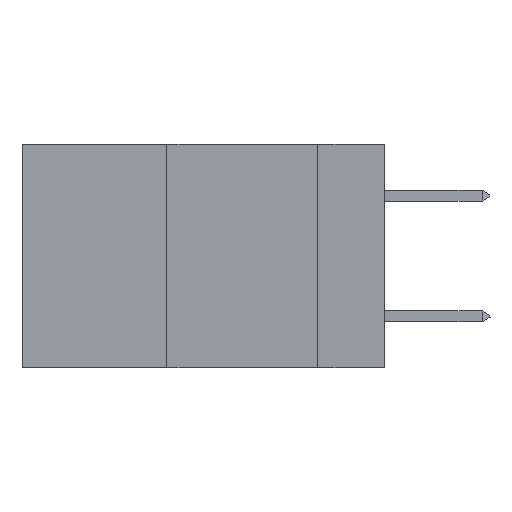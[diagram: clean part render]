
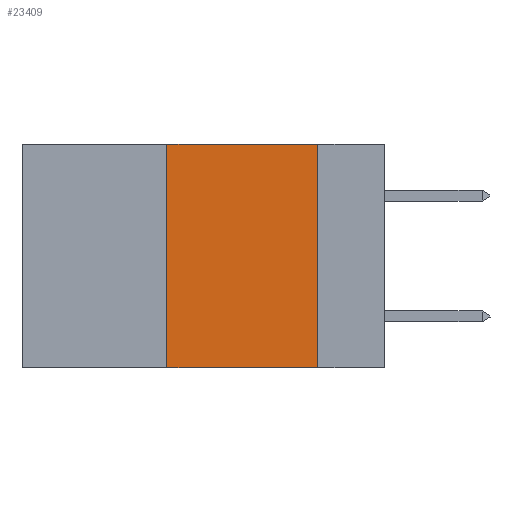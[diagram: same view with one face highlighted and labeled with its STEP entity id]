
A CAD part, left-side view. The second image highlights one B-rep face of the part: STEP entity #23409.
In plain terms, the highlighted planar face has unit normal (-1, 0, 0).
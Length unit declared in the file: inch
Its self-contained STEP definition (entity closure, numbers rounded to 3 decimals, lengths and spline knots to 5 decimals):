
#653 = VECTOR ( 'NONE', #5931, 39.37008 ) ;
#799 = EDGE_CURVE ( 'NONE', #15890, #34650, #15822, .T. ) ;
#1412 = VECTOR ( 'NONE', #30496, 39.37008 ) ;
#1832 = AXIS2_PLACEMENT_3D ( 'NONE', #3975, #17176, #7436 ) ;
#2454 = VECTOR ( 'NONE', #18821, 39.37008 ) ;
#3975 = CARTESIAN_POINT ( 'NONE',  ( 0., 0.6, 0. ) ) ;
#5931 = DIRECTION ( 'NONE',  ( 0., -1., 0. ) ) ;
#7372 = EDGE_LOOP ( 'NONE', ( #39668, #15642, #22414, #37461 ) ) ;
#7436 = DIRECTION ( 'NONE',  ( 0., 0., -1. ) ) ;
#8028 = CARTESIAN_POINT ( 'NONE',  ( 0., 0.36, 0. ) ) ;
#9540 = DIRECTION ( 'NONE',  ( 0., 0., -1. ) ) ;
#11028 = CARTESIAN_POINT ( 'NONE',  ( 0., 0.6, -0.37 ) ) ;
#11912 = VERTEX_POINT ( 'NONE', #25792 ) ;
#13782 = EDGE_CURVE ( 'NONE', #11912, #34650, #27890, .T. ) ;
#14836 = LINE ( 'NONE', #28041, #653 ) ;
#15642 = ORIENTED_EDGE ( 'NONE', *, *, #28495, .F. ) ;
#15822 = LINE ( 'NONE', #35713, #42180 ) ;
#15890 = VERTEX_POINT ( 'NONE', #25129 ) ;
#17176 = DIRECTION ( 'NONE',  ( 1., 0., 0. ) ) ;
#18821 = DIRECTION ( 'NONE',  ( 0., 0., 1. ) ) ;
#22067 = EDGE_CURVE ( 'NONE', #11912, #40888, #24680, .T. ) ;
#22414 = ORIENTED_EDGE ( 'NONE', *, *, #22067, .F. ) ;
#23091 = CARTESIAN_POINT ( 'NONE',  ( 0., 0.36, 0. ) ) ;
#23409 = ADVANCED_FACE ( 'NONE', ( #36854 ), #33621, .F. ) ;
#23598 = CARTESIAN_POINT ( 'NONE',  ( 0., 0.11, -0.37 ) ) ;
#24680 = LINE ( 'NONE', #8028, #2454 ) ;
#25129 = CARTESIAN_POINT ( 'NONE',  ( 0., 0.11, 0. ) ) ;
#25792 = CARTESIAN_POINT ( 'NONE',  ( 0., 0.36, -0.37 ) ) ;
#27890 = LINE ( 'NONE', #11028, #1412 ) ;
#28041 = CARTESIAN_POINT ( 'NONE',  ( 0., 0.6, 0. ) ) ;
#28495 = EDGE_CURVE ( 'NONE', #40888, #15890, #14836, .T. ) ;
#30496 = DIRECTION ( 'NONE',  ( 0., -1., 0. ) ) ;
#33621 = PLANE ( 'NONE',  #1832 ) ;
#34650 = VERTEX_POINT ( 'NONE', #23598 ) ;
#35713 = CARTESIAN_POINT ( 'NONE',  ( 0., 0.11, 0. ) ) ;
#36854 = FACE_OUTER_BOUND ( 'NONE', #7372, .T. ) ;
#37461 = ORIENTED_EDGE ( 'NONE', *, *, #13782, .T. ) ;
#39668 = ORIENTED_EDGE ( 'NONE', *, *, #799, .F. ) ;
#40888 = VERTEX_POINT ( 'NONE', #23091 ) ;
#42180 = VECTOR ( 'NONE', #9540, 39.37008 ) ;
